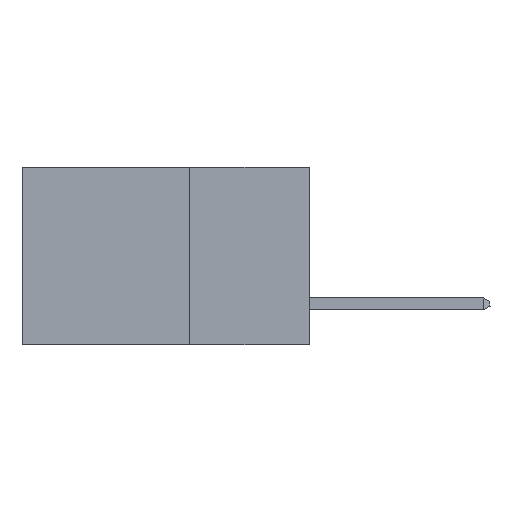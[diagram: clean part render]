
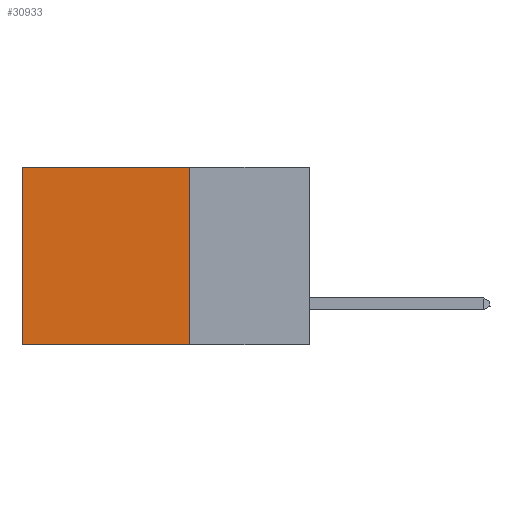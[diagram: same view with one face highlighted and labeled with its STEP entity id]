
A CAD part, left-side view. The second image highlights one B-rep face of the part: STEP entity #30933.
In plain terms, the highlighted planar face has unit normal (-1, 0, 0).
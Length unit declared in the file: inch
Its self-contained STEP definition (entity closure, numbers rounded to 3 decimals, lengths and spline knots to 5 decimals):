
#460 = EDGE_CURVE ( 'NONE', #13898, #45072, #2912, .T. ) ;
#670 = LINE ( 'NONE', #15470, #11477 ) ;
#1201 = PLANE ( 'NONE',  #29013 ) ;
#1353 = DIRECTION ( 'NONE',  ( 0., 1., 0. ) ) ;
#2912 = LINE ( 'NONE', #34337, #16475 ) ;
#3639 = CARTESIAN_POINT ( 'NONE',  ( 0.2875, 0.6, -0.37 ) ) ;
#5904 = ORIENTED_EDGE ( 'NONE', *, *, #41148, .T. ) ;
#9536 = CARTESIAN_POINT ( 'NONE',  ( 0.2875, 0.25, -0.37 ) ) ;
#11163 = CARTESIAN_POINT ( 'NONE',  ( 0.2875, 0.25, 0. ) ) ;
#11477 = VECTOR ( 'NONE', #1353, 39.37008 ) ;
#11870 = VECTOR ( 'NONE', #41923, 39.37008 ) ;
#13898 = VERTEX_POINT ( 'NONE', #9536 ) ;
#14613 = DIRECTION ( 'NONE',  ( 0., 0., -1. ) ) ;
#14726 = LINE ( 'NONE', #46071, #11870 ) ;
#15470 = CARTESIAN_POINT ( 'NONE',  ( 0.2875, 0.25, 0. ) ) ;
#15927 = CARTESIAN_POINT ( 'NONE',  ( 0.2875, 0.25, 0. ) ) ;
#16445 = CARTESIAN_POINT ( 'NONE',  ( 0.2875, 0.6, 0. ) ) ;
#16475 = VECTOR ( 'NONE', #23504, 39.37008 ) ;
#22900 = DIRECTION ( 'NONE',  ( 0., 0., -1. ) ) ;
#23504 = DIRECTION ( 'NONE',  ( 0., 1., 0. ) ) ;
#26312 = EDGE_CURVE ( 'NONE', #40569, #45072, #40848, .T. ) ;
#28119 = ORIENTED_EDGE ( 'NONE', *, *, #26312, .T. ) ;
#28257 = VERTEX_POINT ( 'NONE', #11163 ) ;
#29013 = AXIS2_PLACEMENT_3D ( 'NONE', #15927, #29914, #22900 ) ;
#29914 = DIRECTION ( 'NONE',  ( 1., 0., 0. ) ) ;
#30933 = ADVANCED_FACE ( 'NONE', ( #36068 ), #1201, .F. ) ;
#34337 = CARTESIAN_POINT ( 'NONE',  ( 0.2875, 0.25, -0.37 ) ) ;
#36068 = FACE_OUTER_BOUND ( 'NONE', #42954, .T. ) ;
#36204 = ORIENTED_EDGE ( 'NONE', *, *, #39428, .F. ) ;
#39428 = EDGE_CURVE ( 'NONE', #28257, #13898, #14726, .T. ) ;
#40569 = VERTEX_POINT ( 'NONE', #16445 ) ;
#40848 = LINE ( 'NONE', #43619, #42553 ) ;
#41148 = EDGE_CURVE ( 'NONE', #28257, #40569, #670, .T. ) ;
#41923 = DIRECTION ( 'NONE',  ( 0., 0., -1. ) ) ;
#42553 = VECTOR ( 'NONE', #14613, 39.37008 ) ;
#42576 = ORIENTED_EDGE ( 'NONE', *, *, #460, .F. ) ;
#42954 = EDGE_LOOP ( 'NONE', ( #28119, #42576, #36204, #5904 ) ) ;
#43619 = CARTESIAN_POINT ( 'NONE',  ( 0.2875, 0.6, 0. ) ) ;
#45072 = VERTEX_POINT ( 'NONE', #3639 ) ;
#46071 = CARTESIAN_POINT ( 'NONE',  ( 0.2875, 0.25, 0. ) ) ;
